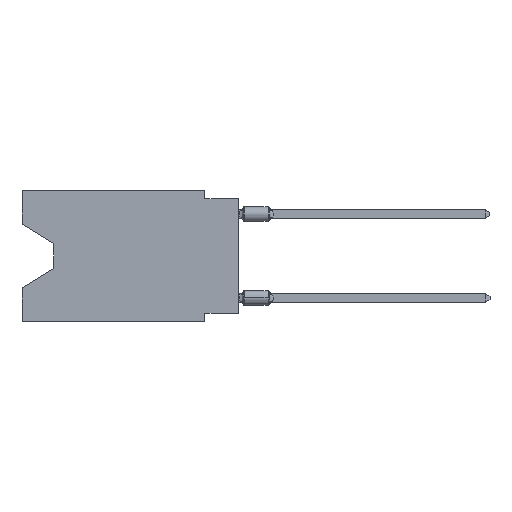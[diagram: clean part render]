
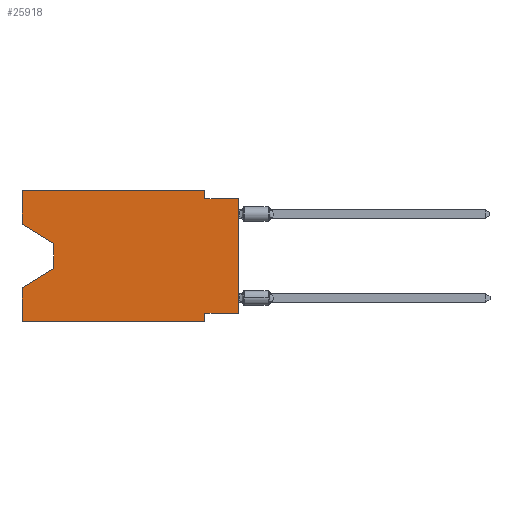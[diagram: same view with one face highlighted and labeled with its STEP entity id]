
A CAD part, left-side view. The second image highlights one B-rep face of the part: STEP entity #25918.
In plain terms, the highlighted planar face has unit normal (-1, 0, 0).
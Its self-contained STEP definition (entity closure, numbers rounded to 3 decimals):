
#540 = LINE ( 'NONE', #3178, #4426 ) ;
#892 = EDGE_CURVE ( 'NONE', #15779, #18747, #12606, .T. ) ;
#1088 = EDGE_CURVE ( 'NONE', #3247, #16280, #6289, .T. ) ;
#1176 = CARTESIAN_POINT ( 'NONE',  ( 0., 2.54, -0.635 ) ) ;
#1374 = VECTOR ( 'NONE', #29689, 1000. ) ;
#1488 = VECTOR ( 'NONE', #24279, 1000. ) ;
#1492 = ORIENTED_EDGE ( 'NONE', *, *, #2665, .F. ) ;
#2535 = VECTOR ( 'NONE', #25620, 1000. ) ;
#2665 = EDGE_CURVE ( 'NONE', #27029, #26269, #7968, .T. ) ;
#2783 = CARTESIAN_POINT ( 'NONE',  ( 0., 0., -0.635 ) ) ;
#2972 = ORIENTED_EDGE ( 'NONE', *, *, #21002, .F. ) ;
#2985 = CARTESIAN_POINT ( 'NONE',  ( 0., 2.54, 0. ) ) ;
#3178 = CARTESIAN_POINT ( 'NONE',  ( 0., 0., 0. ) ) ;
#3247 = VERTEX_POINT ( 'NONE', #23043 ) ;
#3540 = VECTOR ( 'NONE', #5201, 1000. ) ;
#3832 = ORIENTED_EDGE ( 'NONE', *, *, #14529, .F. ) ;
#4112 = CARTESIAN_POINT ( 'NONE',  ( 0., 0., -0.635 ) ) ;
#4426 = VECTOR ( 'NONE', #15372, 1000. ) ;
#5201 = DIRECTION ( 'NONE',  ( 0., 0.855, -0.519 ) ) ;
#5385 = CARTESIAN_POINT ( 'NONE',  ( 0., 16.383, 0. ) ) ;
#6128 = CARTESIAN_POINT ( 'NONE',  ( 0., 16.383, 0. ) ) ;
#6289 = LINE ( 'NONE', #6128, #13491 ) ;
#7913 = VECTOR ( 'NONE', #24190, 1000. ) ;
#7968 = LINE ( 'NONE', #30722, #2535 ) ;
#8857 = LINE ( 'NONE', #31762, #7913 ) ;
#9197 = VECTOR ( 'NONE', #24566, 1000. ) ;
#9556 = CARTESIAN_POINT ( 'NONE',  ( 0., 16.383, -9.906 ) ) ;
#9742 = ORIENTED_EDGE ( 'NONE', *, *, #17574, .F. ) ;
#10701 = EDGE_CURVE ( 'NONE', #28822, #26269, #18052, .T. ) ;
#10967 = LINE ( 'NONE', #26754, #1488 ) ;
#11450 = CARTESIAN_POINT ( 'NONE',  ( 0., 16.383, -7.36 ) ) ;
#11682 = LINE ( 'NONE', #9556, #1374 ) ;
#12606 = LINE ( 'NONE', #19871, #24047 ) ;
#12766 = CARTESIAN_POINT ( 'NONE',  ( 0., 16.383, -2.546 ) ) ;
#13164 = ORIENTED_EDGE ( 'NONE', *, *, #28478, .T. ) ;
#13491 = VECTOR ( 'NONE', #18491, 1000. ) ;
#13822 = ORIENTED_EDGE ( 'NONE', *, *, #14094, .T. ) ;
#14094 = EDGE_CURVE ( 'NONE', #3247, #28626, #20045, .T. ) ;
#14529 = EDGE_CURVE ( 'NONE', #18747, #19641, #22311, .T. ) ;
#14543 = CARTESIAN_POINT ( 'NONE',  ( 0., 2.54, -9.906 ) ) ;
#14685 = EDGE_CURVE ( 'NONE', #15779, #25622, #540, .T. ) ;
#14930 = AXIS2_PLACEMENT_3D ( 'NONE', #5385, #30467, #14939 ) ;
#14939 = DIRECTION ( 'NONE',  ( 0., 0., -1. ) ) ;
#15075 = ORIENTED_EDGE ( 'NONE', *, *, #14685, .T. ) ;
#15080 = DIRECTION ( 'NONE',  ( 0., 1., 0. ) ) ;
#15276 = PLANE ( 'NONE',  #14930 ) ;
#15369 = VECTOR ( 'NONE', #22683, 1000. ) ;
#15372 = DIRECTION ( 'NONE',  ( 0., 0., 1. ) ) ;
#15779 = VERTEX_POINT ( 'NONE', #21993 ) ;
#16280 = VERTEX_POINT ( 'NONE', #27903 ) ;
#16341 = ORIENTED_EDGE ( 'NONE', *, *, #27230, .F. ) ;
#17574 = EDGE_CURVE ( 'NONE', #21008, #18841, #20797, .T. ) ;
#17997 = CARTESIAN_POINT ( 'NONE',  ( 0., 16.383, -9.906 ) ) ;
#18052 = LINE ( 'NONE', #20047, #3540 ) ;
#18491 = DIRECTION ( 'NONE',  ( 0., 0., 1. ) ) ;
#18747 = VERTEX_POINT ( 'NONE', #30410 ) ;
#18841 = VERTEX_POINT ( 'NONE', #1176 ) ;
#19641 = VERTEX_POINT ( 'NONE', #21353 ) ;
#19871 = CARTESIAN_POINT ( 'NONE',  ( 0., 0., -9.271 ) ) ;
#20045 = LINE ( 'NONE', #12766, #15369 ) ;
#20047 = CARTESIAN_POINT ( 'NONE',  ( 0., 13.97, -5.893 ) ) ;
#20160 = DIRECTION ( 'NONE',  ( 0., 0., -1. ) ) ;
#20797 = LINE ( 'NONE', #2985, #26010 ) ;
#21002 = EDGE_CURVE ( 'NONE', #16280, #21008, #8857, .T. ) ;
#21008 = VERTEX_POINT ( 'NONE', #29303 ) ;
#21353 = CARTESIAN_POINT ( 'NONE',  ( 0., 2.54, -9.906 ) ) ;
#21993 = CARTESIAN_POINT ( 'NONE',  ( 0., 0., -9.271 ) ) ;
#22029 = ORIENTED_EDGE ( 'NONE', *, *, #892, .F. ) ;
#22060 = CARTESIAN_POINT ( 'NONE',  ( 0., 13.97, -5.893 ) ) ;
#22311 = LINE ( 'NONE', #14543, #25506 ) ;
#22683 = DIRECTION ( 'NONE',  ( 0., -0.855, -0.519 ) ) ;
#23043 = CARTESIAN_POINT ( 'NONE',  ( 0., 16.383, -2.546 ) ) ;
#23113 = DIRECTION ( 'NONE',  ( 0., 0., -1. ) ) ;
#24047 = VECTOR ( 'NONE', #15080, 1000. ) ;
#24190 = DIRECTION ( 'NONE',  ( 0., -1., 0. ) ) ;
#24247 = LINE ( 'NONE', #4112, #9197 ) ;
#24279 = DIRECTION ( 'NONE',  ( 0., 0., -1. ) ) ;
#24566 = DIRECTION ( 'NONE',  ( 0., -1., 0. ) ) ;
#24612 = EDGE_LOOP ( 'NONE', ( #13822, #31687, #28953, #1492, #13164, #3832, #22029, #15075, #16341, #9742, #2972, #30152 ) ) ;
#25506 = VECTOR ( 'NONE', #20160, 1000. ) ;
#25620 = DIRECTION ( 'NONE',  ( 0., 0., 1. ) ) ;
#25622 = VERTEX_POINT ( 'NONE', #2783 ) ;
#25918 = ADVANCED_FACE ( 'NONE', ( #30140 ), #15276, .F. ) ;
#26010 = VECTOR ( 'NONE', #23113, 1000. ) ;
#26269 = VERTEX_POINT ( 'NONE', #11450 ) ;
#26754 = CARTESIAN_POINT ( 'NONE',  ( 0., 13.97, -4.013 ) ) ;
#27029 = VERTEX_POINT ( 'NONE', #17997 ) ;
#27230 = EDGE_CURVE ( 'NONE', #18841, #25622, #24247, .T. ) ;
#27903 = CARTESIAN_POINT ( 'NONE',  ( 0., 16.383, 0. ) ) ;
#28478 = EDGE_CURVE ( 'NONE', #27029, #19641, #11682, .T. ) ;
#28626 = VERTEX_POINT ( 'NONE', #30185 ) ;
#28822 = VERTEX_POINT ( 'NONE', #22060 ) ;
#28953 = ORIENTED_EDGE ( 'NONE', *, *, #10701, .T. ) ;
#29303 = CARTESIAN_POINT ( 'NONE',  ( 0., 2.54, 0. ) ) ;
#29689 = DIRECTION ( 'NONE',  ( 0., -1., 0. ) ) ;
#30140 = FACE_OUTER_BOUND ( 'NONE', #24612, .T. ) ;
#30152 = ORIENTED_EDGE ( 'NONE', *, *, #1088, .F. ) ;
#30185 = CARTESIAN_POINT ( 'NONE',  ( 0., 13.97, -4.013 ) ) ;
#30410 = CARTESIAN_POINT ( 'NONE',  ( 0., 2.54, -9.271 ) ) ;
#30467 = DIRECTION ( 'NONE',  ( 1., 0., 0. ) ) ;
#30722 = CARTESIAN_POINT ( 'NONE',  ( 0., 16.383, 0. ) ) ;
#31267 = EDGE_CURVE ( 'NONE', #28626, #28822, #10967, .T. ) ;
#31687 = ORIENTED_EDGE ( 'NONE', *, *, #31267, .T. ) ;
#31762 = CARTESIAN_POINT ( 'NONE',  ( 0., 16.383, 0. ) ) ;
